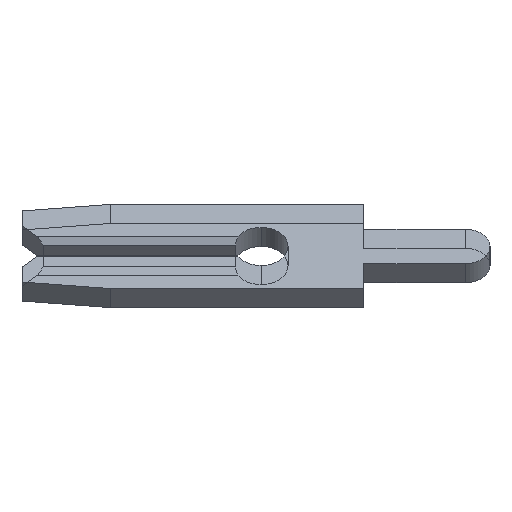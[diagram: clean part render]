
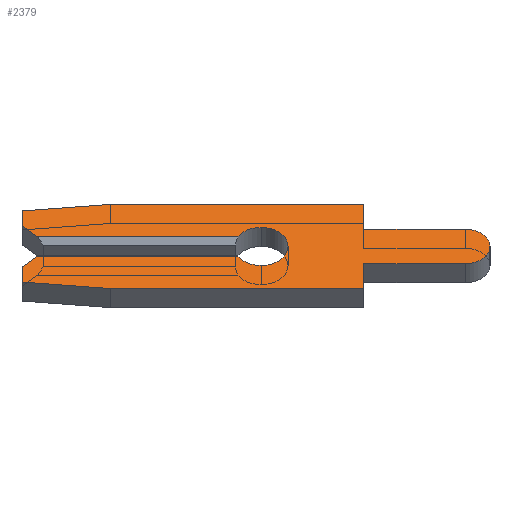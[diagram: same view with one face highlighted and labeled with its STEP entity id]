
A CAD part, left-side view. The second image highlights one B-rep face of the part: STEP entity #2379.
In plain terms, the highlighted face is planar.
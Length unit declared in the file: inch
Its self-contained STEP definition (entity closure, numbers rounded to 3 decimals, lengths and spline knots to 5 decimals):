
#7 = VERTEX_POINT ( 'NONE', #852 ) ;
#15 = VECTOR ( 'NONE', #361, 39.37008 ) ;
#20 = CARTESIAN_POINT ( 'NONE',  ( -0.013, 0.146, -0.0575 ) ) ;
#23 = DIRECTION ( 'NONE',  ( 0., 0., -1. ) ) ;
#38 = CARTESIAN_POINT ( 'NONE',  ( -0.013, 0., 0. ) ) ;
#42 = ORIENTED_EDGE ( 'NONE', *, *, #295, .F. ) ;
#47 = CARTESIAN_POINT ( 'NONE',  ( -0.013, 0., 0. ) ) ;
#90 = VERTEX_POINT ( 'NONE', #1055 ) ;
#92 = CARTESIAN_POINT ( 'NONE',  ( -0.013, 0.146, -0.0575 ) ) ;
#101 = CARTESIAN_POINT ( 'NONE',  ( -0.013, 0.231, 0.013 ) ) ;
#125 = LINE ( 'NONE', #1596, #1927 ) ;
#145 = VECTOR ( 'NONE', #2373, 39.37008 ) ;
#194 = EDGE_CURVE ( 'NONE', #1189, #2222, #1546, .T. ) ;
#201 = ORIENTED_EDGE ( 'NONE', *, *, #903, .F. ) ;
#204 = ORIENTED_EDGE ( 'NONE', *, *, #616, .F. ) ;
#227 = CARTESIAN_POINT ( 'NONE',  ( -0.013, -0.099, 0.0235 ) ) ;
#235 = VERTEX_POINT ( 'NONE', #280 ) ;
#250 = CARTESIAN_POINT ( 'NONE',  ( -0.013, 0.231, -0.04857 ) ) ;
#279 = VECTOR ( 'NONE', #1119, 39.37008 ) ;
#280 = CARTESIAN_POINT ( 'NONE',  ( -0.013, 0.146, 0.0575 ) ) ;
#292 = VERTEX_POINT ( 'NONE', #1696 ) ;
#295 = EDGE_CURVE ( 'NONE', #1909, #90, #565, .T. ) ;
#306 = CIRCLE ( 'NONE', #1890, 0.026 ) ;
#312 = DIRECTION ( 'NONE',  ( 0., -1., 0. ) ) ;
#361 = DIRECTION ( 'NONE',  ( 0., -0.995, 0.105 ) ) ;
#364 = LINE ( 'NONE', #250, #2262 ) ;
#416 = VERTEX_POINT ( 'NONE', #92 ) ;
#419 = VERTEX_POINT ( 'NONE', #692 ) ;
#439 = EDGE_CURVE ( 'NONE', #2183, #1730, #1132, .T. ) ;
#472 = CARTESIAN_POINT ( 'NONE',  ( -0.013, 0.02252, 0.013 ) ) ;
#476 = EDGE_CURVE ( 'NONE', #1880, #419, #1508, .T. ) ;
#546 = ORIENTED_EDGE ( 'NONE', *, *, #710, .F. ) ;
#565 = LINE ( 'NONE', #1925, #279 ) ;
#568 = CARTESIAN_POINT ( 'NONE',  ( -0.013, -0.099, 0.0575 ) ) ;
#572 = EDGE_CURVE ( 'NONE', #2154, #1595, #306, .T. ) ;
#581 = CARTESIAN_POINT ( 'NONE',  ( -0.013, -0.099, -0.0575 ) ) ;
#616 = EDGE_CURVE ( 'NONE', #803, #1189, #1344, .T. ) ;
#647 = CARTESIAN_POINT ( 'NONE',  ( -0.013, -0.1975, 0. ) ) ;
#651 = VERTEX_POINT ( 'NONE', #1959 ) ;
#656 = ORIENTED_EDGE ( 'NONE', *, *, #439, .T. ) ;
#677 = AXIS2_PLACEMENT_3D ( 'NONE', #38, #2059, #862 ) ;
#688 = LINE ( 'NONE', #20, #145 ) ;
#692 = CARTESIAN_POINT ( 'NONE',  ( -0.013, 0.231, 0.04857 ) ) ;
#710 = EDGE_CURVE ( 'NONE', #1372, #7, #1312, .T. ) ;
#739 = ORIENTED_EDGE ( 'NONE', *, *, #572, .F. ) ;
#752 = LINE ( 'NONE', #1992, #15 ) ;
#788 = EDGE_CURVE ( 'NONE', #235, #1207, #1760, .T. ) ;
#803 = VERTEX_POINT ( 'NONE', #1539 ) ;
#850 = ORIENTED_EDGE ( 'NONE', *, *, #1603, .F. ) ;
#852 = CARTESIAN_POINT ( 'NONE',  ( -0.013, -0.1975, 0.0235 ) ) ;
#859 = DIRECTION ( 'NONE',  ( 1., 0., 0. ) ) ;
#862 = DIRECTION ( 'NONE',  ( 0., 0., -1. ) ) ;
#889 = ORIENTED_EDGE ( 'NONE', *, *, #476, .F. ) ;
#899 = ORIENTED_EDGE ( 'NONE', *, *, #2418, .F. ) ;
#903 = EDGE_CURVE ( 'NONE', #2183, #1880, #125, .T. ) ;
#939 = DIRECTION ( 'NONE',  ( 0., 0., -1. ) ) ;
#950 = CARTESIAN_POINT ( 'NONE',  ( -0.013, -0.099, 0.0235 ) ) ;
#983 = CARTESIAN_POINT ( 'NONE',  ( -0.013, 0.216, 0.013 ) ) ;
#984 = EDGE_CURVE ( 'NONE', #419, #235, #752, .T. ) ;
#1001 = CARTESIAN_POINT ( 'NONE',  ( -0.013, -0.099, 0.0575 ) ) ;
#1008 = DIRECTION ( 'NONE',  ( 0., 0.707, 0.707 ) ) ;
#1017 = VECTOR ( 'NONE', #1517, 39.37008 ) ;
#1044 = LINE ( 'NONE', #1833, #2048 ) ;
#1046 = DIRECTION ( 'NONE',  ( 0., 0., 1. ) ) ;
#1055 = CARTESIAN_POINT ( 'NONE',  ( -0.013, -0.099, -0.0235 ) ) ;
#1075 = EDGE_CURVE ( 'NONE', #292, #416, #688, .T. ) ;
#1109 = CARTESIAN_POINT ( 'NONE',  ( -0.013, -0.1975, -0.0235 ) ) ;
#1119 = DIRECTION ( 'NONE',  ( 0., 1., 0. ) ) ;
#1132 = LINE ( 'NONE', #101, #2419 ) ;
#1145 = EDGE_CURVE ( 'NONE', #1207, #1372, #1792, .T. ) ;
#1153 = LINE ( 'NONE', #581, #2113 ) ;
#1176 = ORIENTED_EDGE ( 'NONE', *, *, #1075, .F. ) ;
#1183 = ORIENTED_EDGE ( 'NONE', *, *, #2525, .F. ) ;
#1189 = VERTEX_POINT ( 'NONE', #1789 ) ;
#1207 = VERTEX_POINT ( 'NONE', #1001 ) ;
#1241 = CARTESIAN_POINT ( 'NONE',  ( -0.013, 0., 0. ) ) ;
#1252 = EDGE_CURVE ( 'NONE', #1595, #1730, #1543, .T. ) ;
#1312 = LINE ( 'NONE', #950, #1893 ) ;
#1344 = LINE ( 'NONE', #1346, #1669 ) ;
#1346 = CARTESIAN_POINT ( 'NONE',  ( -0.013, 0.2105, -0.0075 ) ) ;
#1372 = VERTEX_POINT ( 'NONE', #227 ) ;
#1401 = CARTESIAN_POINT ( 'NONE',  ( -0.013, 0., 0. ) ) ;
#1411 = DIRECTION ( 'NONE',  ( 0., 0., -1. ) ) ;
#1460 = CARTESIAN_POINT ( 'NONE',  ( -0.013, 0., 0.026 ) ) ;
#1486 = AXIS2_PLACEMENT_3D ( 'NONE', #647, #859, #2479 ) ;
#1508 = LINE ( 'NONE', #1907, #2486 ) ;
#1514 = EDGE_CURVE ( 'NONE', #7, #1909, #1668, .T. ) ;
#1517 = DIRECTION ( 'NONE',  ( 0., -1., 0. ) ) ;
#1539 = CARTESIAN_POINT ( 'NONE',  ( -0.013, 0.231, -0.028 ) ) ;
#1543 = CIRCLE ( 'NONE', #1900, 0.026 ) ;
#1546 = LINE ( 'NONE', #1897, #1017 ) ;
#1562 = DIRECTION ( 'NONE',  ( -1., 0., 0. ) ) ;
#1570 = CIRCLE ( 'NONE', #677, 0.026 ) ;
#1595 = VERTEX_POINT ( 'NONE', #1460 ) ;
#1596 = CARTESIAN_POINT ( 'NONE',  ( -0.013, 0.2105, 0.0075 ) ) ;
#1603 = EDGE_CURVE ( 'NONE', #416, #651, #364, .T. ) ;
#1646 = EDGE_LOOP ( 'NONE', ( #656, #2013, #739, #1183, #2363, #204, #1687, #850, #1176, #899, #42, #2496, #546, #1818, #1965, #2290, #889, #201 ) ) ;
#1653 = DIRECTION ( 'NONE',  ( 0., 0., -1. ) ) ;
#1668 = CIRCLE ( 'NONE', #1486, 0.0235 ) ;
#1669 = VECTOR ( 'NONE', #2534, 39.37008 ) ;
#1687 = ORIENTED_EDGE ( 'NONE', *, *, #2540, .F. ) ;
#1696 = CARTESIAN_POINT ( 'NONE',  ( -0.013, -0.099, -0.0575 ) ) ;
#1703 = DIRECTION ( 'NONE',  ( 0., 0., 1. ) ) ;
#1707 = CARTESIAN_POINT ( 'NONE',  ( -0.013, 0.231, 0.028 ) ) ;
#1714 = DIRECTION ( 'NONE',  ( 0., -1., 0. ) ) ;
#1730 = VERTEX_POINT ( 'NONE', #472 ) ;
#1760 = LINE ( 'NONE', #2140, #2021 ) ;
#1777 = CARTESIAN_POINT ( 'NONE',  ( -0.013, 0., -0.026 ) ) ;
#1789 = CARTESIAN_POINT ( 'NONE',  ( -0.013, 0.216, -0.013 ) ) ;
#1792 = LINE ( 'NONE', #568, #2319 ) ;
#1818 = ORIENTED_EDGE ( 'NONE', *, *, #1145, .F. ) ;
#1833 = CARTESIAN_POINT ( 'NONE',  ( -0.013, 0.231, -0.028 ) ) ;
#1855 = DIRECTION ( 'NONE',  ( -1., 0., 0. ) ) ;
#1880 = VERTEX_POINT ( 'NONE', #1707 ) ;
#1890 = AXIS2_PLACEMENT_3D ( 'NONE', #1401, #1562, #939 ) ;
#1893 = VECTOR ( 'NONE', #312, 39.37008 ) ;
#1897 = CARTESIAN_POINT ( 'NONE',  ( -0.013, 0., -0.013 ) ) ;
#1900 = AXIS2_PLACEMENT_3D ( 'NONE', #47, #1855, #1411 ) ;
#1907 = CARTESIAN_POINT ( 'NONE',  ( -0.013, 0.231, 0.028 ) ) ;
#1909 = VERTEX_POINT ( 'NONE', #1109 ) ;
#1925 = CARTESIAN_POINT ( 'NONE',  ( -0.013, -0.099, -0.0235 ) ) ;
#1927 = VECTOR ( 'NONE', #1008, 39.37008 ) ;
#1942 = DIRECTION ( 'NONE',  ( 0., -1., 0. ) ) ;
#1959 = CARTESIAN_POINT ( 'NONE',  ( -0.013, 0.231, -0.04857 ) ) ;
#1965 = ORIENTED_EDGE ( 'NONE', *, *, #788, .F. ) ;
#1978 = DIRECTION ( 'NONE',  ( 0., 0., -1. ) ) ;
#1984 = CARTESIAN_POINT ( 'NONE',  ( -0.013, 0.02252, -0.013 ) ) ;
#1992 = CARTESIAN_POINT ( 'NONE',  ( -0.013, 0.231, 0.04857 ) ) ;
#2013 = ORIENTED_EDGE ( 'NONE', *, *, #1252, .F. ) ;
#2021 = VECTOR ( 'NONE', #1942, 39.37008 ) ;
#2027 = DIRECTION ( 'NONE',  ( 1., 0., 0. ) ) ;
#2048 = VECTOR ( 'NONE', #1046, 39.37008 ) ;
#2059 = DIRECTION ( 'NONE',  ( -1., 0., 0. ) ) ;
#2067 = AXIS2_PLACEMENT_3D ( 'NONE', #1241, #2027, #23 ) ;
#2113 = VECTOR ( 'NONE', #1653, 39.37008 ) ;
#2140 = CARTESIAN_POINT ( 'NONE',  ( -0.013, 0.146, 0.0575 ) ) ;
#2154 = VERTEX_POINT ( 'NONE', #1777 ) ;
#2183 = VERTEX_POINT ( 'NONE', #983 ) ;
#2200 = PLANE ( 'NONE',  #2067 ) ;
#2222 = VERTEX_POINT ( 'NONE', #1984 ) ;
#2262 = VECTOR ( 'NONE', #2485, 39.37008 ) ;
#2290 = ORIENTED_EDGE ( 'NONE', *, *, #984, .F. ) ;
#2316 = FACE_OUTER_BOUND ( 'NONE', #1646, .T. ) ;
#2319 = VECTOR ( 'NONE', #1978, 39.37008 ) ;
#2363 = ORIENTED_EDGE ( 'NONE', *, *, #194, .F. ) ;
#2373 = DIRECTION ( 'NONE',  ( 0., 1., 0. ) ) ;
#2379 = ADVANCED_FACE ( 'NONE', ( #2316 ), #2200, .F. ) ;
#2418 = EDGE_CURVE ( 'NONE', #90, #292, #1153, .T. ) ;
#2419 = VECTOR ( 'NONE', #1714, 39.37008 ) ;
#2479 = DIRECTION ( 'NONE',  ( 0., 0., 1. ) ) ;
#2485 = DIRECTION ( 'NONE',  ( 0., 0.995, 0.105 ) ) ;
#2486 = VECTOR ( 'NONE', #1703, 39.37008 ) ;
#2496 = ORIENTED_EDGE ( 'NONE', *, *, #1514, .F. ) ;
#2525 = EDGE_CURVE ( 'NONE', #2222, #2154, #1570, .T. ) ;
#2534 = DIRECTION ( 'NONE',  ( 0., -0.707, 0.707 ) ) ;
#2540 = EDGE_CURVE ( 'NONE', #651, #803, #1044, .T. ) ;
